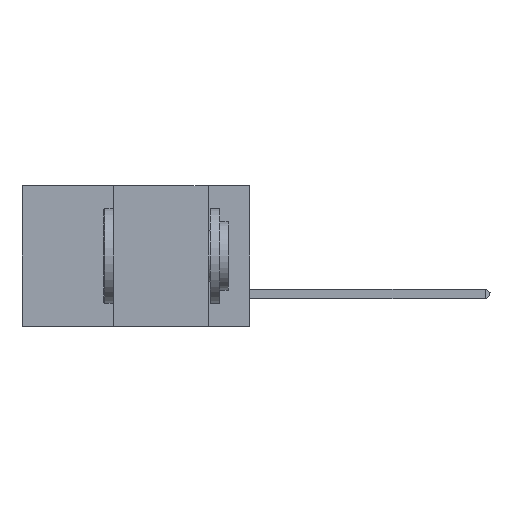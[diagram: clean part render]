
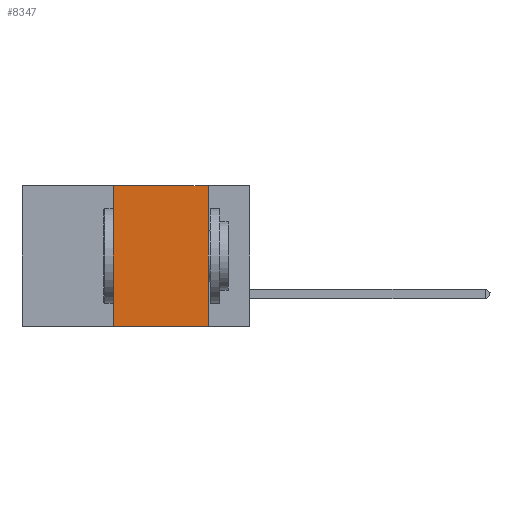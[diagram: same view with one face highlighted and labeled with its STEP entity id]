
A CAD part, left-side view. The second image highlights one B-rep face of the part: STEP entity #8347.
In plain terms, the highlighted planar face has unit normal (-1, 0, 0).
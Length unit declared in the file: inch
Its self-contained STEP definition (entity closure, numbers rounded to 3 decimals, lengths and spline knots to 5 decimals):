
#870 = DIRECTION ( 'NONE',  ( 0., 0., -1. ) ) ;
#1776 = VECTOR ( 'NONE', #12469, 39.37008 ) ;
#2067 = LINE ( 'NONE', #22017, #1776 ) ;
#2170 = VERTEX_POINT ( 'NONE', #21414 ) ;
#2998 = VERTEX_POINT ( 'NONE', #14127 ) ;
#4810 = CARTESIAN_POINT ( 'NONE',  ( 0., 0.6, -0.37 ) ) ;
#4905 = AXIS2_PLACEMENT_3D ( 'NONE', #22007, #20301, #870 ) ;
#6033 = EDGE_LOOP ( 'NONE', ( #12541, #18611, #24280, #19637 ) ) ;
#6814 = PLANE ( 'NONE',  #4905 ) ;
#7377 = LINE ( 'NONE', #14333, #16990 ) ;
#7526 = DIRECTION ( 'NONE',  ( 0., -1., 0. ) ) ;
#8302 = CARTESIAN_POINT ( 'NONE',  ( 0., 0.11, 0. ) ) ;
#8347 = ADVANCED_FACE ( 'NONE', ( #20178 ), #6814, .F. ) ;
#10350 = DIRECTION ( 'NONE',  ( 0., -1., 0. ) ) ;
#11466 = CARTESIAN_POINT ( 'NONE',  ( 0., 0.6, 0. ) ) ;
#12469 = DIRECTION ( 'NONE',  ( 0., 0., -1. ) ) ;
#12541 = ORIENTED_EDGE ( 'NONE', *, *, #23192, .F. ) ;
#13274 = LINE ( 'NONE', #4810, #18093 ) ;
#14127 = CARTESIAN_POINT ( 'NONE',  ( 0., 0.11, -0.37 ) ) ;
#14333 = CARTESIAN_POINT ( 'NONE',  ( 0., 0.36, 0. ) ) ;
#14662 = EDGE_CURVE ( 'NONE', #2170, #2998, #13274, .T. ) ;
#15995 = VERTEX_POINT ( 'NONE', #16732 ) ;
#16732 = CARTESIAN_POINT ( 'NONE',  ( 0., 0.36, 0. ) ) ;
#16879 = VERTEX_POINT ( 'NONE', #8302 ) ;
#16990 = VECTOR ( 'NONE', #20170, 39.37008 ) ;
#17144 = VECTOR ( 'NONE', #7526, 39.37008 ) ;
#18093 = VECTOR ( 'NONE', #10350, 39.37008 ) ;
#18581 = EDGE_CURVE ( 'NONE', #2170, #15995, #7377, .T. ) ;
#18611 = ORIENTED_EDGE ( 'NONE', *, *, #21462, .F. ) ;
#19637 = ORIENTED_EDGE ( 'NONE', *, *, #14662, .T. ) ;
#20170 = DIRECTION ( 'NONE',  ( 0., 0., 1. ) ) ;
#20178 = FACE_OUTER_BOUND ( 'NONE', #6033, .T. ) ;
#20301 = DIRECTION ( 'NONE',  ( 1., 0., 0. ) ) ;
#21414 = CARTESIAN_POINT ( 'NONE',  ( 0., 0.36, -0.37 ) ) ;
#21462 = EDGE_CURVE ( 'NONE', #15995, #16879, #22668, .T. ) ;
#22007 = CARTESIAN_POINT ( 'NONE',  ( 0., 0.6, 0. ) ) ;
#22017 = CARTESIAN_POINT ( 'NONE',  ( 0., 0.11, 0. ) ) ;
#22668 = LINE ( 'NONE', #11466, #17144 ) ;
#23192 = EDGE_CURVE ( 'NONE', #16879, #2998, #2067, .T. ) ;
#24280 = ORIENTED_EDGE ( 'NONE', *, *, #18581, .F. ) ;
